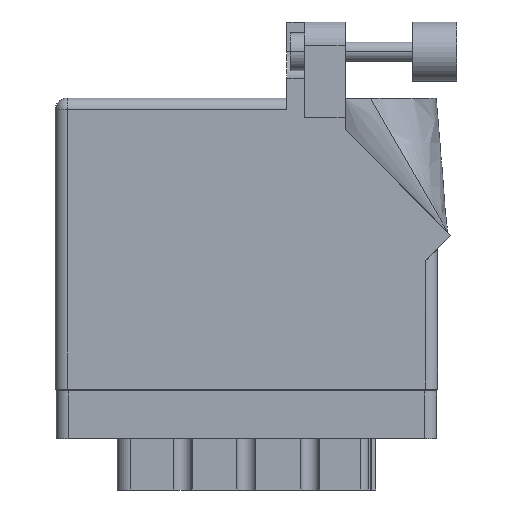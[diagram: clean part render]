
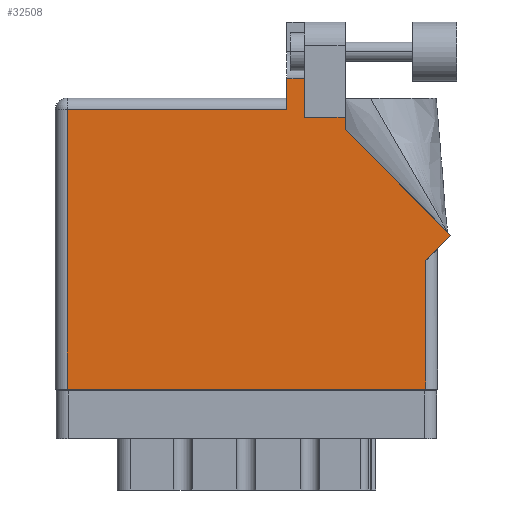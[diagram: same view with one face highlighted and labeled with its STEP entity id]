
A CAD part, front view. The second image highlights one B-rep face of the part: STEP entity #32508.
In plain terms, the highlighted face is planar.
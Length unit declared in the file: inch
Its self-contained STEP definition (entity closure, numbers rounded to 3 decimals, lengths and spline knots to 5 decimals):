
#331 = VECTOR ( 'NONE', #28499, 39.37008 ) ;
#888 = ORIENTED_EDGE ( 'NONE', *, *, #41039, .T. ) ;
#1082 = VERTEX_POINT ( 'NONE', #17518 ) ;
#1438 = ORIENTED_EDGE ( 'NONE', *, *, #15735, .T. ) ;
#1937 = DIRECTION ( 'NONE',  ( -1., 0., 0. ) ) ;
#2389 = VERTEX_POINT ( 'NONE', #37752 ) ;
#2763 = VECTOR ( 'NONE', #22010, 39.37008 ) ;
#2956 = CARTESIAN_POINT ( 'NONE',  ( 1.524, 1.36442, 0. ) ) ;
#3144 = CARTESIAN_POINT ( 'NONE',  ( 0., 1.468, 0. ) ) ;
#4605 = ORIENTED_EDGE ( 'NONE', *, *, #38153, .T. ) ;
#4935 = VERTEX_POINT ( 'NONE', #25394 ) ;
#5634 = ORIENTED_EDGE ( 'NONE', *, *, #37652, .T. ) ;
#6037 = CARTESIAN_POINT ( 'NONE',  ( 1.524, 1.43, 0. ) ) ;
#6212 = LINE ( 'NONE', #15394, #28725 ) ;
#6673 = CARTESIAN_POINT ( 'NONE',  ( 1.311, 1.43, 0. ) ) ;
#6876 = ORIENTED_EDGE ( 'NONE', *, *, #28587, .T. ) ;
#7078 = VERTEX_POINT ( 'NONE', #6037 ) ;
#7782 = VECTOR ( 'NONE', #30675, 39.37008 ) ;
#7998 = EDGE_CURVE ( 'NONE', #20220, #2389, #28788, .T. ) ;
#8271 = DIRECTION ( 'NONE',  ( 0., -1., 0. ) ) ;
#8734 = CARTESIAN_POINT ( 'NONE',  ( 1.217, 1.53, 0. ) ) ;
#8968 = CARTESIAN_POINT ( 'NONE',  ( 1.311, 1.6315, 0. ) ) ;
#9269 = LINE ( 'NONE', #8734, #38832 ) ;
#9798 = LINE ( 'NONE', #2956, #34342 ) ;
#10185 = DIRECTION ( 'NONE',  ( 0., 0., -1. ) ) ;
#10215 = DIRECTION ( 'NONE',  ( 1., 0., 0. ) ) ;
#10326 = VECTOR ( 'NONE', #10215, 39.37008 ) ;
#11171 = VECTOR ( 'NONE', #41571, 39.37008 ) ;
#11310 = EDGE_CURVE ( 'NONE', #2389, #20076, #9269, .T. ) ;
#11790 = CARTESIAN_POINT ( 'NONE',  ( 1.64177, 1.6315, 0. ) ) ;
#12005 = CARTESIAN_POINT ( 'NONE',  ( 0.062, 1.468, 0. ) ) ;
#13218 = LINE ( 'NONE', #6673, #11171 ) ;
#13429 = LINE ( 'NONE', #33619, #22409 ) ;
#13433 = PLANE ( 'NONE',  #36507 ) ;
#14049 = VERTEX_POINT ( 'NONE', #12005 ) ;
#14701 = CARTESIAN_POINT ( 'NONE',  ( 1.524, 1.43, 0. ) ) ;
#15273 = VERTEX_POINT ( 'NONE', #35169 ) ;
#15394 = CARTESIAN_POINT ( 'NONE',  ( 2.01, 0.737, 0. ) ) ;
#15735 = EDGE_CURVE ( 'NONE', #20076, #14049, #25856, .T. ) ;
#16445 = ORIENTED_EDGE ( 'NONE', *, *, #17806, .T. ) ;
#16906 = CARTESIAN_POINT ( 'NONE',  ( 0., 1.53, 0. ) ) ;
#17518 = CARTESIAN_POINT ( 'NONE',  ( 0.062, 0., 0. ) ) ;
#17806 = EDGE_CURVE ( 'NONE', #14049, #1082, #13429, .T. ) ;
#18442 = ORIENTED_EDGE ( 'NONE', *, *, #38723, .T. ) ;
#18554 = ORIENTED_EDGE ( 'NONE', *, *, #19845, .T. ) ;
#18795 = DIRECTION ( 'NONE',  ( 0., 1., 0. ) ) ;
#18806 = LINE ( 'NONE', #38064, #2763 ) ;
#18971 = EDGE_CURVE ( 'NONE', #15273, #7078, #9798, .T. ) ;
#19845 = EDGE_CURVE ( 'NONE', #41478, #20220, #13218, .T. ) ;
#20076 = VERTEX_POINT ( 'NONE', #23573 ) ;
#20220 = VERTEX_POINT ( 'NONE', #8968 ) ;
#20312 = LINE ( 'NONE', #33169, #10326 ) ;
#20361 = LINE ( 'NONE', #21909, #331 ) ;
#21909 = CARTESIAN_POINT ( 'NONE',  ( 2.08071, 0.80771, 0. ) ) ;
#22010 = DIRECTION ( 'NONE',  ( 0., 1., 0. ) ) ;
#22409 = VECTOR ( 'NONE', #8271, 39.37008 ) ;
#23032 = CARTESIAN_POINT ( 'NONE',  ( 1.311, 1.43, 0. ) ) ;
#23573 = CARTESIAN_POINT ( 'NONE',  ( 1.217, 1.468, 0. ) ) ;
#24801 = ORIENTED_EDGE ( 'NONE', *, *, #7998, .T. ) ;
#25291 = ORIENTED_EDGE ( 'NONE', *, *, #11310, .T. ) ;
#25394 = CARTESIAN_POINT ( 'NONE',  ( 1.948, 0.675, 0. ) ) ;
#25527 = DIRECTION ( 'NONE',  ( -1., 0., 0. ) ) ;
#25856 = LINE ( 'NONE', #3144, #37952 ) ;
#26547 = DIRECTION ( 'NONE',  ( -1., 0., 0. ) ) ;
#28499 = DIRECTION ( 'NONE',  ( -0.707, 0.707, 0. ) ) ;
#28587 = EDGE_CURVE ( 'NONE', #4935, #36065, #6212, .T. ) ;
#28725 = VECTOR ( 'NONE', #40909, 39.37008 ) ;
#28788 = LINE ( 'NONE', #11790, #7782 ) ;
#29054 = LINE ( 'NONE', #14701, #32106 ) ;
#30675 = DIRECTION ( 'NONE',  ( -1., 0., 0. ) ) ;
#30797 = CARTESIAN_POINT ( 'NONE',  ( 1.948, 0., 0. ) ) ;
#31676 = CARTESIAN_POINT ( 'NONE',  ( 2.08071, 0.80771, 0. ) ) ;
#32106 = VECTOR ( 'NONE', #1937, 39.37008 ) ;
#32166 = FACE_OUTER_BOUND ( 'NONE', #32552, .T. ) ;
#32508 = ADVANCED_FACE ( 'NONE', ( #32166 ), #13433, .F. ) ;
#32552 = EDGE_LOOP ( 'NONE', ( #18554, #24801, #25291, #1438, #16445, #5634, #18442, #6876, #4605, #39180, #888 ) ) ;
#33169 = CARTESIAN_POINT ( 'NONE',  ( 0., 0., 0. ) ) ;
#33619 = CARTESIAN_POINT ( 'NONE',  ( 0.062, 0., 0. ) ) ;
#33841 = VERTEX_POINT ( 'NONE', #30797 ) ;
#34342 = VECTOR ( 'NONE', #18795, 39.37008 ) ;
#35169 = CARTESIAN_POINT ( 'NONE',  ( 1.524, 1.36442, 0. ) ) ;
#36065 = VERTEX_POINT ( 'NONE', #31676 ) ;
#36507 = AXIS2_PLACEMENT_3D ( 'NONE', #16906, #10185, #26547 ) ;
#37652 = EDGE_CURVE ( 'NONE', #1082, #33841, #20312, .T. ) ;
#37752 = CARTESIAN_POINT ( 'NONE',  ( 1.217, 1.6315, 0. ) ) ;
#37952 = VECTOR ( 'NONE', #25527, 39.37008 ) ;
#38064 = CARTESIAN_POINT ( 'NONE',  ( 1.948, 0.737, 0. ) ) ;
#38153 = EDGE_CURVE ( 'NONE', #36065, #15273, #20361, .T. ) ;
#38723 = EDGE_CURVE ( 'NONE', #33841, #4935, #18806, .T. ) ;
#38832 = VECTOR ( 'NONE', #40693, 39.37008 ) ;
#39180 = ORIENTED_EDGE ( 'NONE', *, *, #18971, .T. ) ;
#40693 = DIRECTION ( 'NONE',  ( 0., -1., 0. ) ) ;
#40909 = DIRECTION ( 'NONE',  ( 0.707, 0.707, 0. ) ) ;
#41039 = EDGE_CURVE ( 'NONE', #7078, #41478, #29054, .T. ) ;
#41478 = VERTEX_POINT ( 'NONE', #23032 ) ;
#41571 = DIRECTION ( 'NONE',  ( 0., 1., 0. ) ) ;
